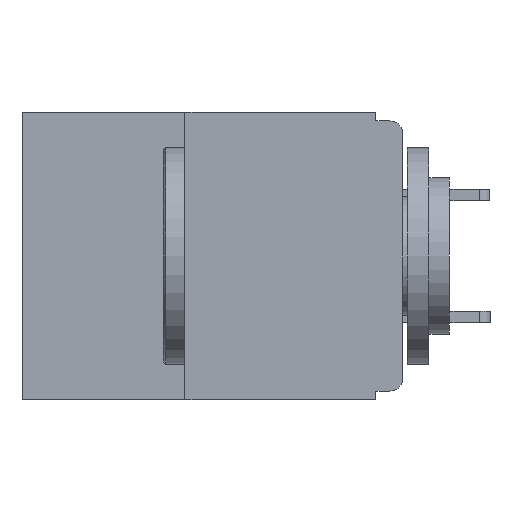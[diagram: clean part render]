
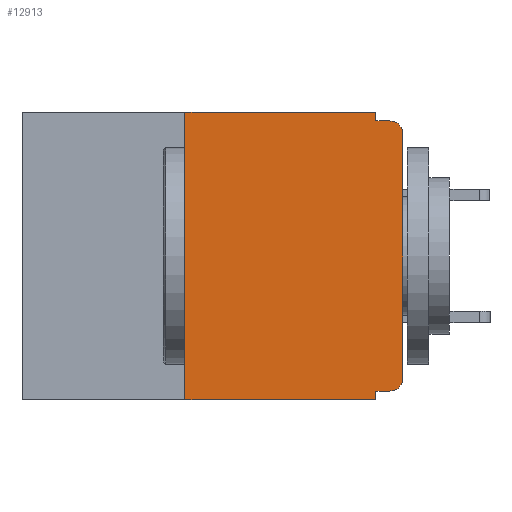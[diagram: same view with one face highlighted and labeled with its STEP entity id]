
A CAD part, left-side view. The second image highlights one B-rep face of the part: STEP entity #12913.
In plain terms, the highlighted planar face has unit normal (-1, 0, 0).
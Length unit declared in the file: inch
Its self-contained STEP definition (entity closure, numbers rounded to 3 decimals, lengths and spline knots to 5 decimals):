
#202 = VERTEX_POINT ( 'NONE', #14427 ) ;
#981 = DIRECTION ( 'NONE',  ( 0., 0., 1. ) ) ;
#1000 = AXIS2_PLACEMENT_3D ( 'NONE', #28262, #11828, #30983 ) ;
#1504 = CARTESIAN_POINT ( 'NONE',  ( 0., 0.031, -0.33 ) ) ;
#3105 = AXIS2_PLACEMENT_3D ( 'NONE', #21280, #7303, #26670 ) ;
#3643 = VERTEX_POINT ( 'NONE', #18020 ) ;
#4559 = EDGE_CURVE ( 'NONE', #35072, #21322, #27906, .T. ) ;
#4614 = EDGE_CURVE ( 'NONE', #7742, #21322, #12471, .T. ) ;
#5009 = ORIENTED_EDGE ( 'NONE', *, *, #10362, .F. ) ;
#6430 = VECTOR ( 'NONE', #981, 39.37008 ) ;
#6502 = CARTESIAN_POINT ( 'NONE',  ( 0., 0.031, 0. ) ) ;
#6573 = CARTESIAN_POINT ( 'NONE',  ( 0., 0.437, 0. ) ) ;
#7101 = ORIENTED_EDGE ( 'NONE', *, *, #9693, .T. ) ;
#7303 = DIRECTION ( 'NONE',  ( 1., 0., 0. ) ) ;
#7560 = AXIS2_PLACEMENT_3D ( 'NONE', #27455, #10998, #30183 ) ;
#7680 = ORIENTED_EDGE ( 'NONE', *, *, #9687, .F. ) ;
#7742 = VERTEX_POINT ( 'NONE', #16892 ) ;
#9077 = ORIENTED_EDGE ( 'NONE', *, *, #35534, .T. ) ;
#9437 = DIRECTION ( 'NONE',  ( 0., -1., 0. ) ) ;
#9530 = ORIENTED_EDGE ( 'NONE', *, *, #25255, .F. ) ;
#9687 = EDGE_CURVE ( 'NONE', #34716, #20783, #22179, .T. ) ;
#9693 = EDGE_CURVE ( 'NONE', #202, #16613, #28526, .T. ) ;
#10362 = EDGE_CURVE ( 'NONE', #25468, #34716, #35185, .T. ) ;
#10434 = ORIENTED_EDGE ( 'NONE', *, *, #4614, .F. ) ;
#10818 = ORIENTED_EDGE ( 'NONE', *, *, #16712, .F. ) ;
#10826 = ORIENTED_EDGE ( 'NONE', *, *, #34316, .T. ) ;
#10998 = DIRECTION ( 'NONE',  ( -1., 0., 0. ) ) ;
#11582 = VECTOR ( 'NONE', #33121, 39.37008 ) ;
#11828 = DIRECTION ( 'NONE',  ( -1., 0., 0. ) ) ;
#12471 = LINE ( 'NONE', #17162, #11582 ) ;
#12478 = CARTESIAN_POINT ( 'NONE',  ( 0., 0.25, -0.33 ) ) ;
#12913 = ADVANCED_FACE ( 'NONE', ( #21577 ), #18521, .F. ) ;
#12980 = CARTESIAN_POINT ( 'NONE',  ( 0., 0.25, -0.33 ) ) ;
#13902 = CARTESIAN_POINT ( 'NONE',  ( 0., 0.25, 0. ) ) ;
#14427 = CARTESIAN_POINT ( 'NONE',  ( 0., 0., -0.305 ) ) ;
#15542 = CARTESIAN_POINT ( 'NONE',  ( 0., 0.031, 0. ) ) ;
#15862 = DIRECTION ( 'NONE',  ( 0., -1., 0. ) ) ;
#15881 = LINE ( 'NONE', #34828, #29482 ) ;
#16613 = VERTEX_POINT ( 'NONE', #31270 ) ;
#16712 = EDGE_CURVE ( 'NONE', #3643, #7742, #24356, .T. ) ;
#16739 = CARTESIAN_POINT ( 'NONE',  ( 0., 0.437, -0.33 ) ) ;
#16892 = CARTESIAN_POINT ( 'NONE',  ( 0., 0.031, -0.32 ) ) ;
#16921 = DIRECTION ( 'NONE',  ( 0., -1., 0. ) ) ;
#17162 = CARTESIAN_POINT ( 'NONE',  ( 0., 0.031, -0.33 ) ) ;
#17163 = VECTOR ( 'NONE', #34428, 39.37008 ) ;
#18020 = CARTESIAN_POINT ( 'NONE',  ( 0., 0.015, -0.32 ) ) ;
#18521 = PLANE ( 'NONE',  #3105 ) ;
#18681 = CIRCLE ( 'NONE', #1000, 0.015 ) ;
#20292 = VERTEX_POINT ( 'NONE', #31285 ) ;
#20524 = DIRECTION ( 'NONE',  ( 0., 0., -1. ) ) ;
#20739 = VECTOR ( 'NONE', #16921, 39.37008 ) ;
#20783 = VERTEX_POINT ( 'NONE', #29066 ) ;
#20864 = VECTOR ( 'NONE', #9437, 39.37008 ) ;
#21280 = CARTESIAN_POINT ( 'NONE',  ( 0., 0.437, 0. ) ) ;
#21322 = VERTEX_POINT ( 'NONE', #1504 ) ;
#21577 = FACE_OUTER_BOUND ( 'NONE', #28663, .T. ) ;
#22179 = LINE ( 'NONE', #6502, #35662 ) ;
#22565 = LINE ( 'NONE', #12980, #28909 ) ;
#22601 = CIRCLE ( 'NONE', #7560, 0.015 ) ;
#23289 = ORIENTED_EDGE ( 'NONE', *, *, #34776, .F. ) ;
#23317 = CARTESIAN_POINT ( 'NONE',  ( 0., 0., 0. ) ) ;
#24356 = LINE ( 'NONE', #29022, #17163 ) ;
#25255 = EDGE_CURVE ( 'NONE', #20783, #20292, #15881, .T. ) ;
#25468 = VERTEX_POINT ( 'NONE', #13902 ) ;
#26670 = DIRECTION ( 'NONE',  ( 0., 0., -1. ) ) ;
#27455 = CARTESIAN_POINT ( 'NONE',  ( 0., 0.015, -0.305 ) ) ;
#27906 = LINE ( 'NONE', #16739, #20739 ) ;
#28262 = CARTESIAN_POINT ( 'NONE',  ( 0., 0.015, -0.025 ) ) ;
#28526 = LINE ( 'NONE', #23317, #6430 ) ;
#28663 = EDGE_LOOP ( 'NONE', ( #7101, #9077, #9530, #7680, #5009, #23289, #33373, #10434, #10818, #10826 ) ) ;
#28909 = VECTOR ( 'NONE', #32059, 39.37008 ) ;
#29022 = CARTESIAN_POINT ( 'NONE',  ( 0., 0., -0.32 ) ) ;
#29066 = CARTESIAN_POINT ( 'NONE',  ( 0., 0.031, -0.01 ) ) ;
#29482 = VECTOR ( 'NONE', #15862, 39.37008 ) ;
#30183 = DIRECTION ( 'NONE',  ( 0., 0., -1. ) ) ;
#30983 = DIRECTION ( 'NONE',  ( 0., 0., -1. ) ) ;
#31270 = CARTESIAN_POINT ( 'NONE',  ( 0., 0., -0.025 ) ) ;
#31285 = CARTESIAN_POINT ( 'NONE',  ( 0., 0.015, -0.01 ) ) ;
#32059 = DIRECTION ( 'NONE',  ( 0., 0., 1. ) ) ;
#33121 = DIRECTION ( 'NONE',  ( 0., 0., -1. ) ) ;
#33373 = ORIENTED_EDGE ( 'NONE', *, *, #4559, .T. ) ;
#34316 = EDGE_CURVE ( 'NONE', #3643, #202, #22601, .T. ) ;
#34428 = DIRECTION ( 'NONE',  ( 0., 1., 0. ) ) ;
#34716 = VERTEX_POINT ( 'NONE', #15542 ) ;
#34776 = EDGE_CURVE ( 'NONE', #35072, #25468, #22565, .T. ) ;
#34828 = CARTESIAN_POINT ( 'NONE',  ( 0., 0., -0.01 ) ) ;
#35072 = VERTEX_POINT ( 'NONE', #12478 ) ;
#35185 = LINE ( 'NONE', #6573, #20864 ) ;
#35534 = EDGE_CURVE ( 'NONE', #16613, #20292, #18681, .T. ) ;
#35662 = VECTOR ( 'NONE', #20524, 39.37008 ) ;
